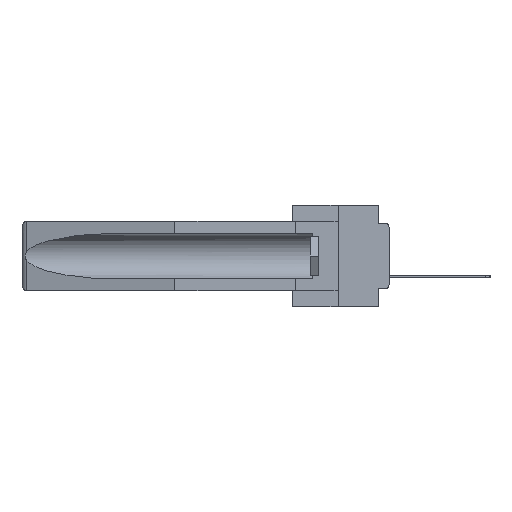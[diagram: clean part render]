
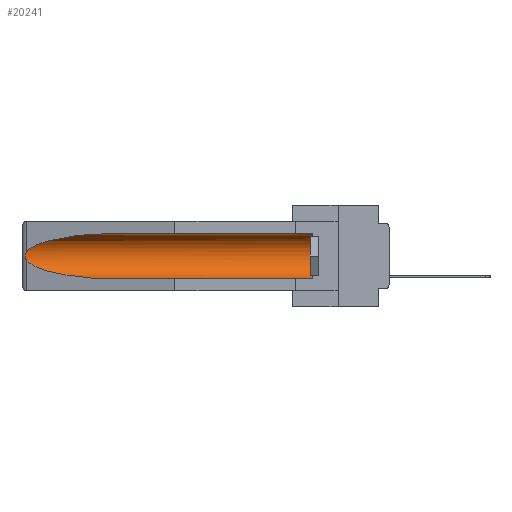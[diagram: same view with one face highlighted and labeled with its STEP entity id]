
A CAD part, left-side view. The second image highlights one B-rep face of the part: STEP entity #20241.
In plain terms, the highlighted cylindrical face has radius 2.857 mm (diameter 5.715 mm), a partial arc.
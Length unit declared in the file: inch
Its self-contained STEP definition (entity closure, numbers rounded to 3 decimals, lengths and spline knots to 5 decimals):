
#650 = VERTEX_POINT ( 'NONE', #14977 ) ;
#1185 = VECTOR ( 'NONE', #29774, 39.37008 ) ;
#1276 = CARTESIAN_POINT ( 'NONE',  ( 0.26537, 1.52718, -0.19328 ) ) ;
#1332 = ORIENTED_EDGE ( 'NONE', *, *, #2974, .T. ) ;
#1597 = CARTESIAN_POINT ( 'NONE',  ( 0.26537, 1.52718, -0.19328 ) ) ;
#1917 = ORIENTED_EDGE ( 'NONE', *, *, #6830, .T. ) ;
#2423 = CARTESIAN_POINT ( 'NONE',  ( 0.2675, 1.53308, -0.17534 ) ) ;
#2974 = EDGE_CURVE ( 'NONE', #15962, #14042, #31168, .T. ) ;
#3106 = ORIENTED_EDGE ( 'NONE', *, *, #15641, .T. ) ;
#3145 =( BOUNDED_CURVE ( )  B_SPLINE_CURVE ( 3, ( #1597, #25272, #30650, #22987 ),
 .UNSPECIFIED., .F., .F. ) 
 B_SPLINE_CURVE_WITH_KNOTS ( ( 4, 4 ),
 ( 0.1948, 1.5708 ),
 .UNSPECIFIED. ) 
 CURVE ( )  GEOMETRIC_REPRESENTATION_ITEM ( )  RATIONAL_B_SPLINE_CURVE ( ( 1., 0.848, 0.848, 1. ) ) 
 REPRESENTATION_ITEM ( '' )  );
#3815 = DIRECTION ( 'NONE',  ( 0., 0., 1. ) ) ;
#4476 = ORIENTED_EDGE ( 'NONE', *, *, #13208, .T. ) ;
#6738 = EDGE_CURVE ( 'NONE', #650, #19012, #30161, .T. ) ;
#6830 = EDGE_CURVE ( 'NONE', #14042, #30358, #17903, .T. ) ;
#7715 = CARTESIAN_POINT ( 'NONE',  ( 0.2675, 1.53308, -0.16763 ) ) ;
#7804 = DIRECTION ( 'NONE',  ( 0., -1., 0. ) ) ;
#7833 = CARTESIAN_POINT ( 'NONE',  ( 0.26537, 1.52718, -0.19328 ) ) ;
#8374 = VECTOR ( 'NONE', #33003, 39.37008 ) ;
#9717 = ORIENTED_EDGE ( 'NONE', *, *, #17201, .T. ) ;
#10230 = CARTESIAN_POINT ( 'NONE',  ( 0.26597, 1.52961, -0.15275 ) ) ;
#10565 = CARTESIAN_POINT ( 'NONE',  ( 0.155, 1.07973, -0.284 ) ) ;
#11305 = VERTEX_POINT ( 'NONE', #1276 ) ;
#12497 = CARTESIAN_POINT ( 'NONE',  ( 0.155, 1.07973, -0.059 ) ) ;
#13208 = EDGE_CURVE ( 'NONE', #650, #15962, #22127, .T. ) ;
#14042 = VERTEX_POINT ( 'NONE', #12497 ) ;
#14613 = FACE_OUTER_BOUND ( 'NONE', #32224, .T. ) ;
#14977 = CARTESIAN_POINT ( 'NONE',  ( 0.155, 0.126, -0.284 ) ) ;
#15641 = EDGE_CURVE ( 'NONE', #11305, #19012, #3145, .T. ) ;
#15962 = VERTEX_POINT ( 'NONE', #29316 ) ;
#17201 = EDGE_CURVE ( 'NONE', #30358, #11305, #31137, .T. ) ;
#17903 =( BOUNDED_CURVE ( )  B_SPLINE_CURVE ( 3, ( #19869, #27314, #22155, #22598 ),
 .UNSPECIFIED., .F., .T. ) 
 B_SPLINE_CURVE_WITH_KNOTS ( ( 4, 4 ),
 ( 4.71239, 6.08839 ),
 .UNSPECIFIED. ) 
 CURVE ( )  GEOMETRIC_REPRESENTATION_ITEM ( )  RATIONAL_B_SPLINE_CURVE ( ( 1., 0.848, 0.848, 1. ) ) 
 REPRESENTATION_ITEM ( '' )  );
#18174 = CARTESIAN_POINT ( 'NONE',  ( 0.2673, 1.5327, -0.16383 ) ) ;
#18376 = CARTESIAN_POINT ( 'NONE',  ( 0.155, 0.126, -0.1715 ) ) ;
#18408 = CARTESIAN_POINT ( 'NONE',  ( 0.26537, 1.52718, -0.14972 ) ) ;
#18625 = AXIS2_PLACEMENT_3D ( 'NONE', #29767, #22211, #3815 ) ;
#18919 = AXIS2_PLACEMENT_3D ( 'NONE', #18376, #7804, #21038 ) ;
#19012 = VERTEX_POINT ( 'NONE', #10565 ) ;
#19869 = CARTESIAN_POINT ( 'NONE',  ( 0.155, 1.07973, -0.059 ) ) ;
#20241 = ADVANCED_FACE ( 'NONE', ( #14613 ), #24873, .F. ) ;
#21038 = DIRECTION ( 'NONE',  ( 0., 0., 1. ) ) ;
#21749 = CARTESIAN_POINT ( 'NONE',  ( 0.155, -0.30754, -0.059 ) ) ;
#22127 = CIRCLE ( 'NONE', #18919, 0.1125 ) ;
#22155 = CARTESIAN_POINT ( 'NONE',  ( 0.25451, 1.48313, -0.09465 ) ) ;
#22211 = DIRECTION ( 'NONE',  ( 0., 1., 0. ) ) ;
#22598 = CARTESIAN_POINT ( 'NONE',  ( 0.26537, 1.52718, -0.14972 ) ) ;
#22987 = CARTESIAN_POINT ( 'NONE',  ( 0.155, 1.07973, -0.284 ) ) ;
#23567 = CARTESIAN_POINT ( 'NONE',  ( 0.26597, 1.5296, -0.19026 ) ) ;
#24223 = ORIENTED_EDGE ( 'NONE', *, *, #6738, .F. ) ;
#24873 = CYLINDRICAL_SURFACE ( 'NONE', #18625, 0.1125 ) ;
#25272 = CARTESIAN_POINT ( 'NONE',  ( 0.25451, 1.48313, -0.24835 ) ) ;
#26081 = CARTESIAN_POINT ( 'NONE',  ( 0.2673, 1.53269, -0.17917 ) ) ;
#26483 = CARTESIAN_POINT ( 'NONE',  ( 0.26537, 1.52718, -0.14972 ) ) ;
#27314 = CARTESIAN_POINT ( 'NONE',  ( 0.21114, 1.30732, -0.059 ) ) ;
#29316 = CARTESIAN_POINT ( 'NONE',  ( 0.155, 0.126, -0.059 ) ) ;
#29767 = CARTESIAN_POINT ( 'NONE',  ( 0.155, -0.30754, -0.1715 ) ) ;
#29774 = DIRECTION ( 'NONE',  ( 0., 1., 0. ) ) ;
#30161 = LINE ( 'NONE', #30176, #8374 ) ;
#30176 = CARTESIAN_POINT ( 'NONE',  ( 0.155, -0.30754, -0.284 ) ) ;
#30358 = VERTEX_POINT ( 'NONE', #26483 ) ;
#30650 = CARTESIAN_POINT ( 'NONE',  ( 0.21114, 1.30732, -0.284 ) ) ;
#31137 = B_SPLINE_CURVE_WITH_KNOTS ( 'NONE', 3,
 ( #18408, #10230, #31240, #18174, #7715, #2423, #26081, #33979, #23567, #7833 ),
 .UNSPECIFIED., .F., .F.,
 ( 4, 2, 2, 2, 4 ),
 ( 0., 0.00029, 0.00058, 0.00087, 0.00117 ),
 .UNSPECIFIED. ) ;
#31168 = LINE ( 'NONE', #21749, #1185 ) ;
#31240 = CARTESIAN_POINT ( 'NONE',  ( 0.26654, 1.53092, -0.15636 ) ) ;
#32224 = EDGE_LOOP ( 'NONE', ( #1917, #9717, #3106, #24223, #4476, #1332 ) ) ;
#33003 = DIRECTION ( 'NONE',  ( 0., 1., 0. ) ) ;
#33979 = CARTESIAN_POINT ( 'NONE',  ( 0.26655, 1.53094, -0.18657 ) ) ;
